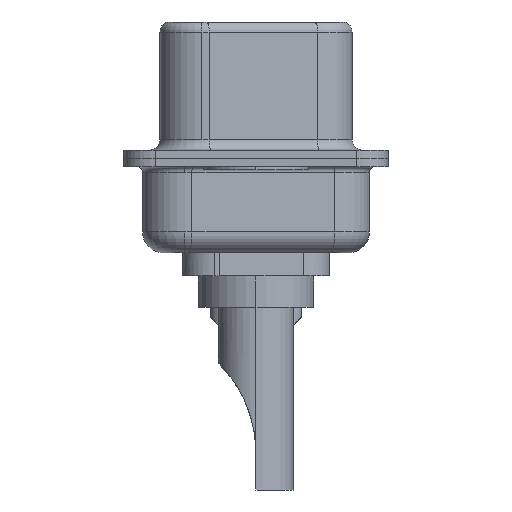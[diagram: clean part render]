
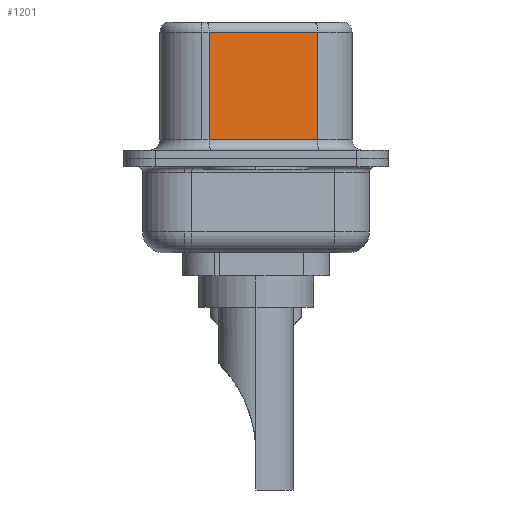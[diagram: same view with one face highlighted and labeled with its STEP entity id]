
A CAD part, left-side view. The second image highlights one B-rep face of the part: STEP entity #1201.
In plain terms, the highlighted planar face has unit normal (-0.985, -0.174, 0).
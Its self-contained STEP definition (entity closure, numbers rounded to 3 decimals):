
#104 = CARTESIAN_POINT ( 'NONE',  ( 4.585, -2.927, 6.02 ) ) ;
#1201 = ADVANCED_FACE ( 'NONE', ( #14149 ), #2163, .F. ) ;
#1245 = VECTOR ( 'NONE', #9367, 1000. ) ;
#1772 = VERTEX_POINT ( 'NONE', #14568 ) ;
#2163 = PLANE ( 'NONE',  #16708 ) ;
#2445 = CARTESIAN_POINT ( 'NONE',  ( 3.675, 2.233, 6.52 ) ) ;
#2801 = ORIENTED_EDGE ( 'NONE', *, *, #8834, .T. ) ;
#2821 = DIRECTION ( 'NONE',  ( 0.174, -0.985, 0. ) ) ;
#3362 = VECTOR ( 'NONE', #2821, 1000. ) ;
#4910 = LINE ( 'NONE', #2445, #14834 ) ;
#5252 = VERTEX_POINT ( 'NONE', #15679 ) ;
#5368 = VERTEX_POINT ( 'NONE', #13446 ) ;
#5954 = CARTESIAN_POINT ( 'NONE',  ( 4.585, -2.927, 0.9 ) ) ;
#6155 = VECTOR ( 'NONE', #16409, 1000. ) ;
#6496 = EDGE_CURVE ( 'NONE', #5252, #5368, #4910, .T. ) ;
#7402 = LINE ( 'NONE', #16669, #6155 ) ;
#7413 = EDGE_CURVE ( 'NONE', #1772, #8625, #7402, .T. ) ;
#7509 = LINE ( 'NONE', #104, #1245 ) ;
#8625 = VERTEX_POINT ( 'NONE', #5954 ) ;
#8834 = EDGE_CURVE ( 'NONE', #5368, #8625, #9988, .T. ) ;
#9367 = DIRECTION ( 'NONE',  ( -0.174, 0.985, 0. ) ) ;
#9988 = LINE ( 'NONE', #11868, #3362 ) ;
#10064 = ORIENTED_EDGE ( 'NONE', *, *, #7413, .F. ) ;
#10164 = ORIENTED_EDGE ( 'NONE', *, *, #11282, .T. ) ;
#11078 = ORIENTED_EDGE ( 'NONE', *, *, #6496, .T. ) ;
#11282 = EDGE_CURVE ( 'NONE', #1772, #5252, #7509, .T. ) ;
#11868 = CARTESIAN_POINT ( 'NONE',  ( 4.585, -2.927, 0.9 ) ) ;
#12819 = CARTESIAN_POINT ( 'NONE',  ( 4.585, -2.927, 6.52 ) ) ;
#13446 = CARTESIAN_POINT ( 'NONE',  ( 3.675, 2.233, 0.9 ) ) ;
#13573 = DIRECTION ( 'NONE',  ( 0., 0., -1. ) ) ;
#14149 = FACE_OUTER_BOUND ( 'NONE', #14200, .T. ) ;
#14200 = EDGE_LOOP ( 'NONE', ( #10064, #10164, #11078, #2801 ) ) ;
#14568 = CARTESIAN_POINT ( 'NONE',  ( 4.585, -2.927, 6.02 ) ) ;
#14834 = VECTOR ( 'NONE', #13573, 1000. ) ;
#15679 = CARTESIAN_POINT ( 'NONE',  ( 3.675, 2.233, 6.02 ) ) ;
#15891 = DIRECTION ( 'NONE',  ( 0.985, 0.174, 0. ) ) ;
#16409 = DIRECTION ( 'NONE',  ( 0., 0., -1. ) ) ;
#16669 = CARTESIAN_POINT ( 'NONE',  ( 4.585, -2.927, 6.52 ) ) ;
#16708 = AXIS2_PLACEMENT_3D ( 'NONE', #12819, #15891, #16776 ) ;
#16776 = DIRECTION ( 'NONE',  ( -0.174, 0.985, 0. ) ) ;
